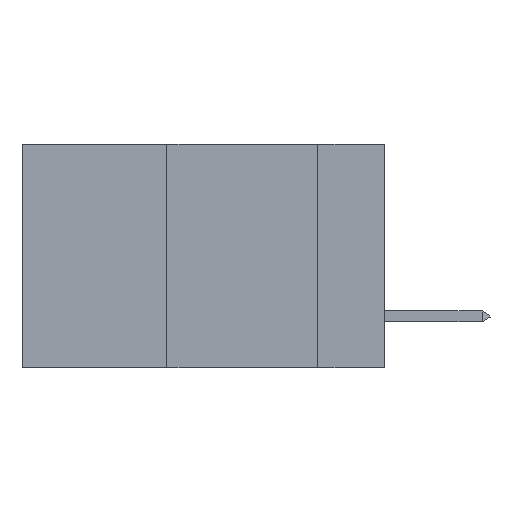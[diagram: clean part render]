
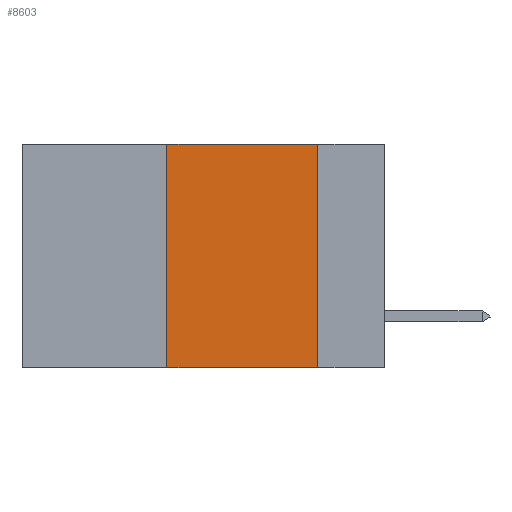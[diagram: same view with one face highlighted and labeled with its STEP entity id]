
A CAD part, left-side view. The second image highlights one B-rep face of the part: STEP entity #8603.
In plain terms, the highlighted planar face has unit normal (-1, 0, 0).
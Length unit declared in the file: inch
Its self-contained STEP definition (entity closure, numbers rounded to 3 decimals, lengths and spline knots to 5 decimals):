
#908 = FACE_OUTER_BOUND ( 'NONE', #17082, .T. ) ;
#1096 = EDGE_CURVE ( 'NONE', #5083, #15592, #18615, .T. ) ;
#1360 = ORIENTED_EDGE ( 'NONE', *, *, #1096, .F. ) ;
#2508 = DIRECTION ( 'NONE',  ( 1., 0., 0. ) ) ;
#4254 = VECTOR ( 'NONE', #19300, 39.37008 ) ;
#5083 = VERTEX_POINT ( 'NONE', #14447 ) ;
#7263 = CARTESIAN_POINT ( 'NONE',  ( 0., 0.11, 0. ) ) ;
#8603 = ADVANCED_FACE ( 'NONE', ( #908 ), #20481, .F. ) ;
#8791 = EDGE_CURVE ( 'NONE', #16706, #9893, #14003, .T. ) ;
#9381 = EDGE_CURVE ( 'NONE', #15592, #9893, #13713, .T. ) ;
#9388 = CARTESIAN_POINT ( 'NONE',  ( 0., 0.6, -0.37 ) ) ;
#9893 = VERTEX_POINT ( 'NONE', #19086 ) ;
#10022 = LINE ( 'NONE', #13730, #20060 ) ;
#10237 = ORIENTED_EDGE ( 'NONE', *, *, #17863, .F. ) ;
#12310 = AXIS2_PLACEMENT_3D ( 'NONE', #12318, #2508, #18734 ) ;
#12318 = CARTESIAN_POINT ( 'NONE',  ( 0., 0.6, 0. ) ) ;
#13713 = LINE ( 'NONE', #18518, #17325 ) ;
#13730 = CARTESIAN_POINT ( 'NONE',  ( 0., 0.36, 0. ) ) ;
#14003 = LINE ( 'NONE', #9388, #4254 ) ;
#14116 = ORIENTED_EDGE ( 'NONE', *, *, #9381, .F. ) ;
#14246 = VECTOR ( 'NONE', #16602, 39.37008 ) ;
#14447 = CARTESIAN_POINT ( 'NONE',  ( 0., 0.36, 0. ) ) ;
#15155 = CARTESIAN_POINT ( 'NONE',  ( 0., 0.36, -0.37 ) ) ;
#15592 = VERTEX_POINT ( 'NONE', #7263 ) ;
#16602 = DIRECTION ( 'NONE',  ( 0., -1., 0. ) ) ;
#16608 = DIRECTION ( 'NONE',  ( 0., 0., -1. ) ) ;
#16706 = VERTEX_POINT ( 'NONE', #15155 ) ;
#17082 = EDGE_LOOP ( 'NONE', ( #14116, #1360, #10237, #18403 ) ) ;
#17325 = VECTOR ( 'NONE', #16608, 39.37008 ) ;
#17863 = EDGE_CURVE ( 'NONE', #16706, #5083, #10022, .T. ) ;
#18403 = ORIENTED_EDGE ( 'NONE', *, *, #8791, .T. ) ;
#18518 = CARTESIAN_POINT ( 'NONE',  ( 0., 0.11, 0. ) ) ;
#18615 = LINE ( 'NONE', #19761, #14246 ) ;
#18734 = DIRECTION ( 'NONE',  ( 0., 0., -1. ) ) ;
#19086 = CARTESIAN_POINT ( 'NONE',  ( 0., 0.11, -0.37 ) ) ;
#19300 = DIRECTION ( 'NONE',  ( 0., -1., 0. ) ) ;
#19761 = CARTESIAN_POINT ( 'NONE',  ( 0., 0.6, 0. ) ) ;
#20060 = VECTOR ( 'NONE', #20296, 39.37008 ) ;
#20296 = DIRECTION ( 'NONE',  ( 0., 0., 1. ) ) ;
#20481 = PLANE ( 'NONE',  #12310 ) ;
